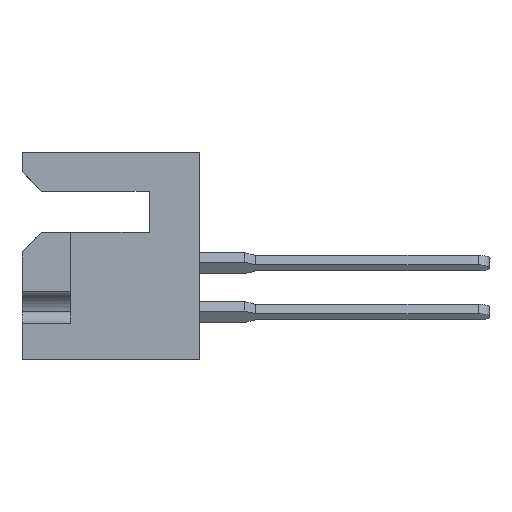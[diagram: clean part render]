
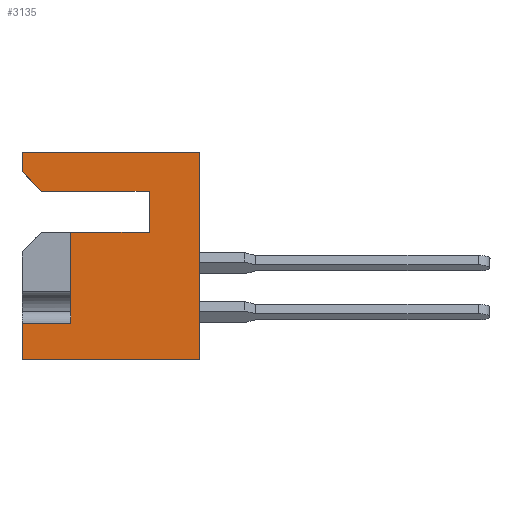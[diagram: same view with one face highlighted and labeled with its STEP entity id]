
A CAD part, left-side view. The second image highlights one B-rep face of the part: STEP entity #3135.
In plain terms, the highlighted planar face has unit normal (-1, 0, 0).
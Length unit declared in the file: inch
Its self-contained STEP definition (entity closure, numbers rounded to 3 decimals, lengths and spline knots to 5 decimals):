
#180 = CARTESIAN_POINT ( 'NONE',  ( 0., 0.453, -0.437 ) ) ;
#228 = CARTESIAN_POINT ( 'NONE',  ( 0., 0.403, -0.1 ) ) ;
#252 = VERTEX_POINT ( 'NONE', #15397 ) ;
#281 = EDGE_LOOP ( 'NONE', ( #4051, #9666, #6124, #15983, #4874, #1629, #13118, #12096, #10693, #722, #4386 ) ) ;
#426 = VECTOR ( 'NONE', #4982, 39.37008 ) ;
#722 = ORIENTED_EDGE ( 'NONE', *, *, #9507, .T. ) ;
#1119 = EDGE_CURVE ( 'NONE', #12865, #7625, #13471, .T. ) ;
#1155 = VECTOR ( 'NONE', #2423, 39.37008 ) ;
#1171 = LINE ( 'NONE', #2398, #11318 ) ;
#1365 = DIRECTION ( 'NONE',  ( 1., 0., 0. ) ) ;
#1429 = VECTOR ( 'NONE', #12366, 39.37008 ) ;
#1629 = ORIENTED_EDGE ( 'NONE', *, *, #6149, .F. ) ;
#1851 = CARTESIAN_POINT ( 'NONE',  ( 0., 0.403, -0.1 ) ) ;
#2119 = CARTESIAN_POINT ( 'NONE',  ( 0., 0.128, -0.205 ) ) ;
#2285 = VECTOR ( 'NONE', #10199, 39.37008 ) ;
#2398 = CARTESIAN_POINT ( 'NONE',  ( 0., 0.128, -0.1 ) ) ;
#2423 = DIRECTION ( 'NONE',  ( 0., -1., 0. ) ) ;
#2601 = CARTESIAN_POINT ( 'NONE',  ( 0., 0.453, -0.05 ) ) ;
#2604 = LINE ( 'NONE', #1851, #10341 ) ;
#3021 = CARTESIAN_POINT ( 'NONE',  ( 0., 0.453, -0.531 ) ) ;
#3121 = CARTESIAN_POINT ( 'NONE',  ( 0., 0., -0.531 ) ) ;
#3135 = ADVANCED_FACE ( 'NONE', ( #10407 ), #8092, .F. ) ;
#3240 = DIRECTION ( 'NONE',  ( 0., 0., -1. ) ) ;
#3306 = CARTESIAN_POINT ( 'NONE',  ( 0., 0.328, -0.205 ) ) ;
#3419 = DIRECTION ( 'NONE',  ( 0., -1., 0. ) ) ;
#3473 = LINE ( 'NONE', #8962, #4463 ) ;
#3793 = LINE ( 'NONE', #9873, #426 ) ;
#3950 = AXIS2_PLACEMENT_3D ( 'NONE', #7851, #1365, #3240 ) ;
#3990 = LINE ( 'NONE', #3021, #13134 ) ;
#4051 = ORIENTED_EDGE ( 'NONE', *, *, #15599, .T. ) ;
#4386 = ORIENTED_EDGE ( 'NONE', *, *, #8471, .F. ) ;
#4427 = CARTESIAN_POINT ( 'NONE',  ( 0., 0.328, -0.205 ) ) ;
#4463 = VECTOR ( 'NONE', #15121, 39.37008 ) ;
#4874 = ORIENTED_EDGE ( 'NONE', *, *, #12040, .F. ) ;
#4982 = DIRECTION ( 'NONE',  ( 0., 0., 1. ) ) ;
#4994 = LINE ( 'NONE', #7614, #1429 ) ;
#6007 = VERTEX_POINT ( 'NONE', #16003 ) ;
#6054 = CARTESIAN_POINT ( 'NONE',  ( 0., 0.453, -0.531 ) ) ;
#6124 = ORIENTED_EDGE ( 'NONE', *, *, #6525, .T. ) ;
#6149 = EDGE_CURVE ( 'NONE', #13107, #6007, #3793, .T. ) ;
#6302 = VECTOR ( 'NONE', #10652, 39.37008 ) ;
#6525 = EDGE_CURVE ( 'NONE', #12865, #15792, #3990, .T. ) ;
#7593 = EDGE_CURVE ( 'NONE', #252, #14937, #1171, .T. ) ;
#7614 = CARTESIAN_POINT ( 'NONE',  ( 0., 0.328, -0.437 ) ) ;
#7625 = VERTEX_POINT ( 'NONE', #180 ) ;
#7647 = VECTOR ( 'NONE', #12456, 39.37008 ) ;
#7688 = CARTESIAN_POINT ( 'NONE',  ( 0., 0., 0. ) ) ;
#7851 = CARTESIAN_POINT ( 'NONE',  ( 0., 0.453, 0. ) ) ;
#8092 = PLANE ( 'NONE',  #3950 ) ;
#8278 = LINE ( 'NONE', #4427, #6302 ) ;
#8471 = EDGE_CURVE ( 'NONE', #14006, #14690, #8278, .T. ) ;
#8962 = CARTESIAN_POINT ( 'NONE',  ( 0., 0.128, -0.1 ) ) ;
#9079 = VECTOR ( 'NONE', #9461, 39.37008 ) ;
#9461 = DIRECTION ( 'NONE',  ( 0., 0., 1. ) ) ;
#9507 = EDGE_CURVE ( 'NONE', #252, #14690, #11654, .T. ) ;
#9642 = CARTESIAN_POINT ( 'NONE',  ( 0., 0.128, -0.1 ) ) ;
#9666 = ORIENTED_EDGE ( 'NONE', *, *, #1119, .F. ) ;
#9873 = CARTESIAN_POINT ( 'NONE',  ( 0., 0.453, 0. ) ) ;
#10199 = DIRECTION ( 'NONE',  ( 0., 0., 1. ) ) ;
#10220 = EDGE_CURVE ( 'NONE', #14937, #16266, #3473, .T. ) ;
#10297 = EDGE_CURVE ( 'NONE', #15792, #15027, #12820, .T. ) ;
#10341 = VECTOR ( 'NONE', #12018, 39.37008 ) ;
#10407 = FACE_OUTER_BOUND ( 'NONE', #281, .T. ) ;
#10652 = DIRECTION ( 'NONE',  ( 0., 0., 1. ) ) ;
#10693 = ORIENTED_EDGE ( 'NONE', *, *, #7593, .F. ) ;
#10704 = CARTESIAN_POINT ( 'NONE',  ( 0., 0.453, 0. ) ) ;
#11318 = VECTOR ( 'NONE', #12418, 39.37008 ) ;
#11654 = LINE ( 'NONE', #2119, #7647 ) ;
#12018 = DIRECTION ( 'NONE',  ( 0., -0.707, -0.707 ) ) ;
#12040 = EDGE_CURVE ( 'NONE', #6007, #15027, #13281, .T. ) ;
#12096 = ORIENTED_EDGE ( 'NONE', *, *, #10220, .F. ) ;
#12366 = DIRECTION ( 'NONE',  ( 0., 1., 0. ) ) ;
#12418 = DIRECTION ( 'NONE',  ( 0., 0., 1. ) ) ;
#12456 = DIRECTION ( 'NONE',  ( 0., 1., 0. ) ) ;
#12763 = CARTESIAN_POINT ( 'NONE',  ( 0., 0.453, 0. ) ) ;
#12820 = LINE ( 'NONE', #7688, #2285 ) ;
#12865 = VERTEX_POINT ( 'NONE', #6054 ) ;
#13012 = CARTESIAN_POINT ( 'NONE',  ( 0., 0.328, -0.437 ) ) ;
#13107 = VERTEX_POINT ( 'NONE', #2601 ) ;
#13118 = ORIENTED_EDGE ( 'NONE', *, *, #15790, .T. ) ;
#13134 = VECTOR ( 'NONE', #3419, 39.37008 ) ;
#13281 = LINE ( 'NONE', #12763, #1155 ) ;
#13471 = LINE ( 'NONE', #10704, #9079 ) ;
#14006 = VERTEX_POINT ( 'NONE', #13012 ) ;
#14690 = VERTEX_POINT ( 'NONE', #3306 ) ;
#14749 = CARTESIAN_POINT ( 'NONE',  ( 0., 0., 0. ) ) ;
#14937 = VERTEX_POINT ( 'NONE', #9642 ) ;
#15027 = VERTEX_POINT ( 'NONE', #14749 ) ;
#15121 = DIRECTION ( 'NONE',  ( 0., 1., 0. ) ) ;
#15397 = CARTESIAN_POINT ( 'NONE',  ( 0., 0.128, -0.205 ) ) ;
#15599 = EDGE_CURVE ( 'NONE', #14006, #7625, #4994, .T. ) ;
#15790 = EDGE_CURVE ( 'NONE', #13107, #16266, #2604, .T. ) ;
#15792 = VERTEX_POINT ( 'NONE', #3121 ) ;
#15983 = ORIENTED_EDGE ( 'NONE', *, *, #10297, .T. ) ;
#16003 = CARTESIAN_POINT ( 'NONE',  ( 0., 0.453, 0. ) ) ;
#16266 = VERTEX_POINT ( 'NONE', #228 ) ;
